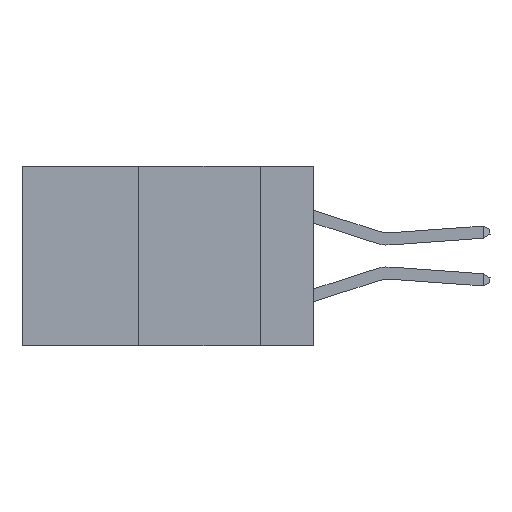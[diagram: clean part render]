
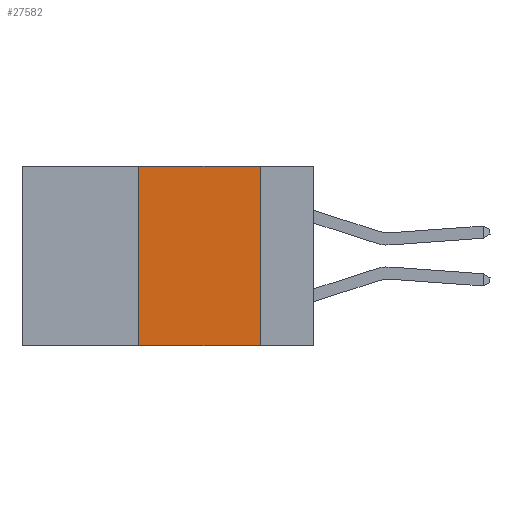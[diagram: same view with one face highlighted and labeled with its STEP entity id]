
A CAD part, left-side view. The second image highlights one B-rep face of the part: STEP entity #27582.
In plain terms, the highlighted planar face has unit normal (-1, 0, 0).
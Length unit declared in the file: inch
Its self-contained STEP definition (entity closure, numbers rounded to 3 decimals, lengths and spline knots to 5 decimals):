
#554 = LINE ( 'NONE', #28562, #16769 ) ;
#2205 = LINE ( 'NONE', #9405, #35292 ) ;
#2295 = CARTESIAN_POINT ( 'NONE',  ( 0., 0.6, 0. ) ) ;
#4300 = LINE ( 'NONE', #18743, #19579 ) ;
#4423 = CARTESIAN_POINT ( 'NONE',  ( 0., 0.36, 0. ) ) ;
#4455 = CARTESIAN_POINT ( 'NONE',  ( 0., 0.36, 0. ) ) ;
#4985 = CARTESIAN_POINT ( 'NONE',  ( 0., 0.11, -0.37 ) ) ;
#6189 = EDGE_LOOP ( 'NONE', ( #34086, #7446, #6768, #28198 ) ) ;
#6768 = ORIENTED_EDGE ( 'NONE', *, *, #27265, .F. ) ;
#7446 = ORIENTED_EDGE ( 'NONE', *, *, #34490, .F. ) ;
#7625 = VERTEX_POINT ( 'NONE', #4985 ) ;
#8143 = VERTEX_POINT ( 'NONE', #9642 ) ;
#8358 = PLANE ( 'NONE',  #26035 ) ;
#8622 = DIRECTION ( 'NONE',  ( 0., 0., -1. ) ) ;
#9405 = CARTESIAN_POINT ( 'NONE',  ( 0., 0.6, -0.37 ) ) ;
#9642 = CARTESIAN_POINT ( 'NONE',  ( 0., 0.11, 0. ) ) ;
#9791 = DIRECTION ( 'NONE',  ( 0., -1., 0. ) ) ;
#14366 = DIRECTION ( 'NONE',  ( 1., 0., 0. ) ) ;
#14879 = VERTEX_POINT ( 'NONE', #4455 ) ;
#16769 = VECTOR ( 'NONE', #8622, 39.37008 ) ;
#18743 = CARTESIAN_POINT ( 'NONE',  ( 0., 0.6, 0. ) ) ;
#19312 = DIRECTION ( 'NONE',  ( 0., 0., 1. ) ) ;
#19579 = VECTOR ( 'NONE', #9791, 39.37008 ) ;
#21915 = VECTOR ( 'NONE', #19312, 39.37008 ) ;
#26035 = AXIS2_PLACEMENT_3D ( 'NONE', #2295, #14366, #29098 ) ;
#27265 = EDGE_CURVE ( 'NONE', #27794, #14879, #36777, .T. ) ;
#27447 = FACE_OUTER_BOUND ( 'NONE', #6189, .T. ) ;
#27582 = ADVANCED_FACE ( 'NONE', ( #27447 ), #8358, .F. ) ;
#27794 = VERTEX_POINT ( 'NONE', #29987 ) ;
#28198 = ORIENTED_EDGE ( 'NONE', *, *, #37196, .T. ) ;
#28562 = CARTESIAN_POINT ( 'NONE',  ( 0., 0.11, 0. ) ) ;
#28682 = EDGE_CURVE ( 'NONE', #8143, #7625, #554, .T. ) ;
#29098 = DIRECTION ( 'NONE',  ( 0., 0., -1. ) ) ;
#29987 = CARTESIAN_POINT ( 'NONE',  ( 0., 0.36, -0.37 ) ) ;
#30120 = DIRECTION ( 'NONE',  ( 0., -1., 0. ) ) ;
#34086 = ORIENTED_EDGE ( 'NONE', *, *, #28682, .F. ) ;
#34490 = EDGE_CURVE ( 'NONE', #14879, #8143, #4300, .T. ) ;
#35292 = VECTOR ( 'NONE', #30120, 39.37008 ) ;
#36777 = LINE ( 'NONE', #4423, #21915 ) ;
#37196 = EDGE_CURVE ( 'NONE', #27794, #7625, #2205, .T. ) ;
